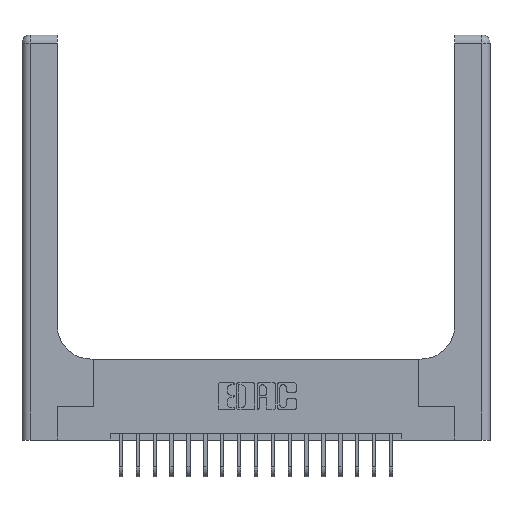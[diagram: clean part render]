
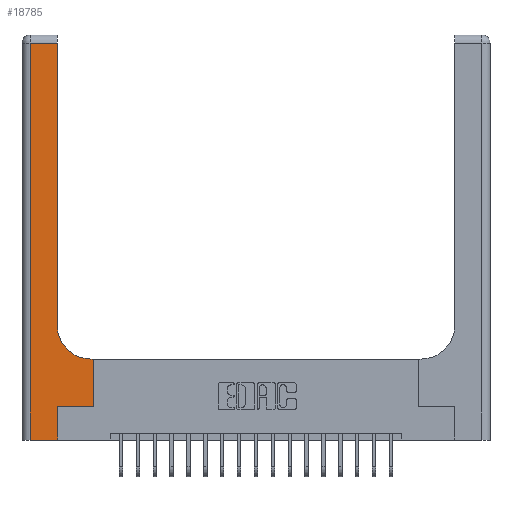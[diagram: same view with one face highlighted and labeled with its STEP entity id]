
A CAD part, top view. The second image highlights one B-rep face of the part: STEP entity #18785.
In plain terms, the highlighted planar face has unit normal (0, 0, 1).
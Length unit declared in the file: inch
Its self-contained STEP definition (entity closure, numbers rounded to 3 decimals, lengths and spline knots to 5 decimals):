
#51 = VERTEX_POINT ( 'NONE', #596 ) ;
#81 = DIRECTION ( 'NONE',  ( 0., 0., -1. ) ) ;
#313 = ORIENTED_EDGE ( 'NONE', *, *, #13694, .T. ) ;
#437 = CARTESIAN_POINT ( 'NONE',  ( 0.265, 0.25, 0.37 ) ) ;
#596 = CARTESIAN_POINT ( 'NONE',  ( 0.528, 0.6, 0.37 ) ) ;
#831 = CARTESIAN_POINT ( 'NONE',  ( 0.26, 3., 0.37 ) ) ;
#1275 = CARTESIAN_POINT ( 'NONE',  ( 0.06, 2.94, 0.37 ) ) ;
#1686 = CARTESIAN_POINT ( 'NONE',  ( 0.06, 3., 0.37 ) ) ;
#1875 = EDGE_CURVE ( 'NONE', #7817, #9303, #14705, .T. ) ;
#2250 = DIRECTION ( 'NONE',  ( 0., 0., -1. ) ) ;
#2325 = DIRECTION ( 'NONE',  ( -1., 0., 0. ) ) ;
#2392 = EDGE_LOOP ( 'NONE', ( #313, #19242, #7877, #4671, #11325, #13675, #17673, #6637, #16897 ) ) ;
#2592 = VECTOR ( 'NONE', #13805, 39.37008 ) ;
#2745 = CARTESIAN_POINT ( 'NONE',  ( 0.265, 0., 0.37 ) ) ;
#2772 = DIRECTION ( 'NONE',  ( 1., 0., 0. ) ) ;
#3063 = CARTESIAN_POINT ( 'NONE',  ( 0.265, 0., 0.37 ) ) ;
#3137 = CARTESIAN_POINT ( 'NONE',  ( 0.528, 0.25, 0.37 ) ) ;
#3657 = VECTOR ( 'NONE', #2325, 39.37008 ) ;
#3799 = EDGE_CURVE ( 'NONE', #13206, #11861, #14245, .T. ) ;
#3817 = DIRECTION ( 'NONE',  ( 0., 1., 0. ) ) ;
#4384 = VERTEX_POINT ( 'NONE', #1275 ) ;
#4571 = VECTOR ( 'NONE', #10963, 39.37008 ) ;
#4671 = ORIENTED_EDGE ( 'NONE', *, *, #13057, .T. ) ;
#4900 = LINE ( 'NONE', #831, #7385 ) ;
#5133 = FACE_OUTER_BOUND ( 'NONE', #2392, .T. ) ;
#5238 = PLANE ( 'NONE',  #5339 ) ;
#5339 = AXIS2_PLACEMENT_3D ( 'NONE', #11292, #2250, #6636 ) ;
#6573 = VERTEX_POINT ( 'NONE', #15112 ) ;
#6621 = CARTESIAN_POINT ( 'NONE',  ( 0.528, 0.25, 0.37 ) ) ;
#6636 = DIRECTION ( 'NONE',  ( -1., 0., 0. ) ) ;
#6637 = ORIENTED_EDGE ( 'NONE', *, *, #12386, .T. ) ;
#7253 = VECTOR ( 'NONE', #18060, 39.37008 ) ;
#7385 = VECTOR ( 'NONE', #3817, 39.37008 ) ;
#7817 = VERTEX_POINT ( 'NONE', #9729 ) ;
#7877 = ORIENTED_EDGE ( 'NONE', *, *, #12841, .T. ) ;
#7968 = VECTOR ( 'NONE', #2772, 39.37008 ) ;
#8030 = VERTEX_POINT ( 'NONE', #16757 ) ;
#9034 = CARTESIAN_POINT ( 'NONE',  ( 0.51, 0.85, 0.37 ) ) ;
#9303 = VERTEX_POINT ( 'NONE', #10813 ) ;
#9430 = VERTEX_POINT ( 'NONE', #2745 ) ;
#9729 = CARTESIAN_POINT ( 'NONE',  ( 0.51, 0.6, 0.37 ) ) ;
#10418 = CARTESIAN_POINT ( 'NONE',  ( 0., 0., 0.37 ) ) ;
#10813 = CARTESIAN_POINT ( 'NONE',  ( 0.26, 0.85, 0.37 ) ) ;
#10963 = DIRECTION ( 'NONE',  ( 1., 0., 0. ) ) ;
#11292 = CARTESIAN_POINT ( 'NONE',  ( 0., 3., 0.37 ) ) ;
#11325 = ORIENTED_EDGE ( 'NONE', *, *, #15930, .T. ) ;
#11861 = VERTEX_POINT ( 'NONE', #6621 ) ;
#12300 = DIRECTION ( 'NONE',  ( 1., 0., 0. ) ) ;
#12336 = LINE ( 'NONE', #18386, #18422 ) ;
#12386 = EDGE_CURVE ( 'NONE', #51, #7817, #12336, .T. ) ;
#12841 = EDGE_CURVE ( 'NONE', #4384, #6573, #15284, .T. ) ;
#13057 = EDGE_CURVE ( 'NONE', #6573, #9430, #16382, .T. ) ;
#13206 = VERTEX_POINT ( 'NONE', #13683 ) ;
#13675 = ORIENTED_EDGE ( 'NONE', *, *, #3799, .T. ) ;
#13683 = CARTESIAN_POINT ( 'NONE',  ( 0.265, 0.25, 0.37 ) ) ;
#13694 = EDGE_CURVE ( 'NONE', #9303, #8030, #4900, .T. ) ;
#13805 = DIRECTION ( 'NONE',  ( 0., -1., 0. ) ) ;
#14245 = LINE ( 'NONE', #437, #4571 ) ;
#14587 = EDGE_CURVE ( 'NONE', #11861, #51, #16942, .T. ) ;
#14705 = CIRCLE ( 'NONE', #19133, 0.25 ) ;
#15112 = CARTESIAN_POINT ( 'NONE',  ( 0.06, 0., 0.37 ) ) ;
#15153 = DIRECTION ( 'NONE',  ( 0., 1., 0. ) ) ;
#15284 = LINE ( 'NONE', #1686, #2592 ) ;
#15362 = LINE ( 'NONE', #3063, #7253 ) ;
#15930 = EDGE_CURVE ( 'NONE', #9430, #13206, #15362, .T. ) ;
#15931 = CARTESIAN_POINT ( 'NONE',  ( 0., 2.94, 0.37 ) ) ;
#16382 = LINE ( 'NONE', #10418, #7968 ) ;
#16757 = CARTESIAN_POINT ( 'NONE',  ( 0.26, 2.94, 0.37 ) ) ;
#16897 = ORIENTED_EDGE ( 'NONE', *, *, #1875, .T. ) ;
#16942 = LINE ( 'NONE', #3137, #17217 ) ;
#17217 = VECTOR ( 'NONE', #15153, 39.37008 ) ;
#17673 = ORIENTED_EDGE ( 'NONE', *, *, #14587, .T. ) ;
#18060 = DIRECTION ( 'NONE',  ( 0., 1., 0. ) ) ;
#18386 = CARTESIAN_POINT ( 'NONE',  ( 0.26, 0.6, 0.37 ) ) ;
#18422 = VECTOR ( 'NONE', #18486, 39.37008 ) ;
#18486 = DIRECTION ( 'NONE',  ( -1., 0., 0. ) ) ;
#18785 = ADVANCED_FACE ( 'NONE', ( #5133 ), #5238, .F. ) ;
#18998 = LINE ( 'NONE', #15931, #3657 ) ;
#19133 = AXIS2_PLACEMENT_3D ( 'NONE', #9034, #81, #12300 ) ;
#19242 = ORIENTED_EDGE ( 'NONE', *, *, #19399, .T. ) ;
#19399 = EDGE_CURVE ( 'NONE', #8030, #4384, #18998, .T. ) ;
